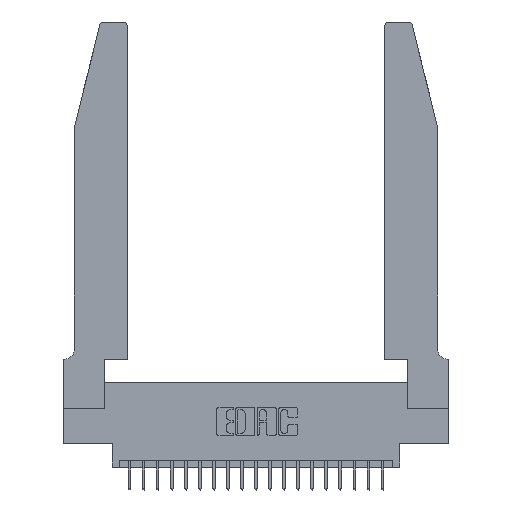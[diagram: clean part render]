
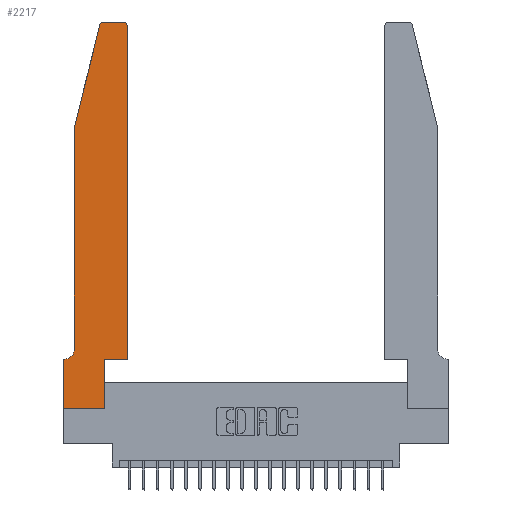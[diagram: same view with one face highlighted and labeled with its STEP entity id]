
A CAD part, top view. The second image highlights one B-rep face of the part: STEP entity #2217.
In plain terms, the highlighted planar face has unit normal (0, 0, 1).
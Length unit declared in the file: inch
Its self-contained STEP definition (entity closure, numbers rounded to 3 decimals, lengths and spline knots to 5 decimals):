
#366 = AXIS2_PLACEMENT_3D ( 'NONE', #951, #13572, #2839 ) ;
#370 = DIRECTION ( 'NONE',  ( 0., 0., 1. ) ) ;
#448 = DIRECTION ( 'NONE',  ( 1., 0., 0. ) ) ;
#672 = AXIS2_PLACEMENT_3D ( 'NONE', #13556, #13503, #14729 ) ;
#673 = CARTESIAN_POINT ( 'NONE',  ( 0.2605, 2.75, 0.37 ) ) ;
#951 = CARTESIAN_POINT ( 'NONE',  ( 0.284, 2.72, 0.37 ) ) ;
#1084 = CARTESIAN_POINT ( 'NONE',  ( 0., 0., 0.37 ) ) ;
#1435 = DIRECTION ( 'NONE',  ( -0.239, -0.971, 0. ) ) ;
#1570 = EDGE_CURVE ( 'NONE', #16445, #22062, #2657, .T. ) ;
#1905 = VERTEX_POINT ( 'NONE', #22014 ) ;
#2094 = VERTEX_POINT ( 'NONE', #20002 ) ;
#2128 = VECTOR ( 'NONE', #18183, 39.37008 ) ;
#2217 = ADVANCED_FACE ( 'NONE', ( #22222 ), #6320, .T. ) ;
#2657 = CIRCLE ( 'NONE', #672, 0.07 ) ;
#2692 = VERTEX_POINT ( 'NONE', #19089 ) ;
#2839 = DIRECTION ( 'NONE',  ( 1., 0., 0. ) ) ;
#3621 = ORIENTED_EDGE ( 'NONE', *, *, #7316, .T. ) ;
#3948 = LINE ( 'NONE', #4196, #8200 ) ;
#4111 = VERTEX_POINT ( 'NONE', #16670 ) ;
#4196 = CARTESIAN_POINT ( 'NONE',  ( 0.0755, 0.35, 0.37 ) ) ;
#4227 = VECTOR ( 'NONE', #13228, 39.37008 ) ;
#4696 = AXIS2_PLACEMENT_3D ( 'NONE', #6292, #370, #448 ) ;
#4809 = VERTEX_POINT ( 'NONE', #1084 ) ;
#5247 = ORIENTED_EDGE ( 'NONE', *, *, #15779, .T. ) ;
#5584 = ORIENTED_EDGE ( 'NONE', *, *, #10149, .T. ) ;
#5890 = DIRECTION ( 'NONE',  ( 0., 0., 1. ) ) ;
#6292 = CARTESIAN_POINT ( 'NONE',  ( 0., 0.35, 0.37 ) ) ;
#6320 = PLANE ( 'NONE',  #4696 ) ;
#6355 = CARTESIAN_POINT ( 'NONE',  ( 0.0755, 2., 0.37 ) ) ;
#6480 = VECTOR ( 'NONE', #13443, 39.37008 ) ;
#6486 = VECTOR ( 'NONE', #14765, 39.37008 ) ;
#6601 = VERTEX_POINT ( 'NONE', #20425 ) ;
#6678 = LINE ( 'NONE', #6851, #20157 ) ;
#6851 = CARTESIAN_POINT ( 'NONE',  ( 0.0755, 2., 0.37 ) ) ;
#7224 = EDGE_CURVE ( 'NONE', #2692, #4111, #15934, .T. ) ;
#7316 = EDGE_CURVE ( 'NONE', #4809, #15855, #13201, .T. ) ;
#7604 = CARTESIAN_POINT ( 'NONE',  ( 0.0055, 0.35, 0.37 ) ) ;
#7618 = CARTESIAN_POINT ( 'NONE',  ( 0.4505, 0.35, 0.37 ) ) ;
#7626 = CARTESIAN_POINT ( 'NONE',  ( 0.2865, 0.35, 0.37 ) ) ;
#7932 = ORIENTED_EDGE ( 'NONE', *, *, #18672, .T. ) ;
#8144 = CARTESIAN_POINT ( 'NONE',  ( 0., 0., 0.37 ) ) ;
#8200 = VECTOR ( 'NONE', #14974, 39.37008 ) ;
#8673 = VECTOR ( 'NONE', #13306, 39.37008 ) ;
#8937 = ORIENTED_EDGE ( 'NONE', *, *, #15851, .T. ) ;
#9087 = VERTEX_POINT ( 'NONE', #16814 ) ;
#9242 = LINE ( 'NONE', #6355, #12320 ) ;
#9661 = CARTESIAN_POINT ( 'NONE',  ( 0., 0., 0.37 ) ) ;
#9767 = EDGE_CURVE ( 'NONE', #6601, #10785, #15601, .T. ) ;
#9821 = EDGE_LOOP ( 'NONE', ( #22665, #20917, #5584, #7932, #10237, #5247, #8937, #3621, #18649, #22607, #12321, #15636 ) ) ;
#10149 = EDGE_CURVE ( 'NONE', #9087, #1905, #6678, .T. ) ;
#10237 = ORIENTED_EDGE ( 'NONE', *, *, #1570, .T. ) ;
#10383 = EDGE_CURVE ( 'NONE', #15855, #2692, #16363, .T. ) ;
#10785 = VERTEX_POINT ( 'NONE', #19156 ) ;
#11072 = VECTOR ( 'NONE', #18880, 39.37008 ) ;
#12320 = VECTOR ( 'NONE', #20446, 39.37008 ) ;
#12321 = ORIENTED_EDGE ( 'NONE', *, *, #13778, .T. ) ;
#13201 = LINE ( 'NONE', #9661, #4227 ) ;
#13228 = DIRECTION ( 'NONE',  ( 1., 0., 0. ) ) ;
#13256 = CARTESIAN_POINT ( 'NONE',  ( 0.0755, 0.42, 0.37 ) ) ;
#13306 = DIRECTION ( 'NONE',  ( -1., 0., 0. ) ) ;
#13443 = DIRECTION ( 'NONE',  ( 0., -1., 0. ) ) ;
#13503 = DIRECTION ( 'NONE',  ( 0., 0., -1. ) ) ;
#13556 = CARTESIAN_POINT ( 'NONE',  ( 0.0055, 0.42, 0.37 ) ) ;
#13572 = DIRECTION ( 'NONE',  ( 0., 0., 1. ) ) ;
#13778 = EDGE_CURVE ( 'NONE', #4111, #6601, #20346, .T. ) ;
#14729 = DIRECTION ( 'NONE',  ( -1., 0., 0. ) ) ;
#14765 = DIRECTION ( 'NONE',  ( 1., 0., 0. ) ) ;
#14974 = DIRECTION ( 'NONE',  ( -1., 0., 0. ) ) ;
#15601 = CIRCLE ( 'NONE', #19499, 0.03 ) ;
#15636 = ORIENTED_EDGE ( 'NONE', *, *, #9767, .T. ) ;
#15779 = EDGE_CURVE ( 'NONE', #22062, #22305, #3948, .T. ) ;
#15851 = EDGE_CURVE ( 'NONE', #22305, #4809, #16458, .T. ) ;
#15855 = VERTEX_POINT ( 'NONE', #22141 ) ;
#15934 = LINE ( 'NONE', #7618, #6486 ) ;
#16363 = LINE ( 'NONE', #7626, #2128 ) ;
#16445 = VERTEX_POINT ( 'NONE', #13256 ) ;
#16458 = LINE ( 'NONE', #8144, #6480 ) ;
#16537 = CARTESIAN_POINT ( 'NONE',  ( 0.4205, 2.72, 0.37 ) ) ;
#16670 = CARTESIAN_POINT ( 'NONE',  ( 0.4505, 0.35, 0.37 ) ) ;
#16814 = CARTESIAN_POINT ( 'NONE',  ( 0.25487, 2.72718, 0.37 ) ) ;
#17148 = CARTESIAN_POINT ( 'NONE',  ( 0.4505, 0.35, 0.37 ) ) ;
#18183 = DIRECTION ( 'NONE',  ( 0., 1., 0. ) ) ;
#18286 = DIRECTION ( 'NONE',  ( 1., 0., 0. ) ) ;
#18649 = ORIENTED_EDGE ( 'NONE', *, *, #10383, .T. ) ;
#18672 = EDGE_CURVE ( 'NONE', #1905, #16445, #9242, .T. ) ;
#18880 = DIRECTION ( 'NONE',  ( 0., 1., 0. ) ) ;
#19089 = CARTESIAN_POINT ( 'NONE',  ( 0.2865, 0.35, 0.37 ) ) ;
#19107 = EDGE_CURVE ( 'NONE', #10785, #2094, #22054, .T. ) ;
#19156 = CARTESIAN_POINT ( 'NONE',  ( 0.4205, 2.75, 0.37 ) ) ;
#19499 = AXIS2_PLACEMENT_3D ( 'NONE', #16537, #5890, #18286 ) ;
#20002 = CARTESIAN_POINT ( 'NONE',  ( 0.284, 2.75, 0.37 ) ) ;
#20157 = VECTOR ( 'NONE', #1435, 39.37008 ) ;
#20346 = LINE ( 'NONE', #17148, #11072 ) ;
#20418 = CARTESIAN_POINT ( 'NONE',  ( 0., 0.35, 0.37 ) ) ;
#20425 = CARTESIAN_POINT ( 'NONE',  ( 0.4505, 2.72, 0.37 ) ) ;
#20446 = DIRECTION ( 'NONE',  ( 0., -1., 0. ) ) ;
#20917 = ORIENTED_EDGE ( 'NONE', *, *, #21181, .T. ) ;
#21139 = CIRCLE ( 'NONE', #366, 0.03 ) ;
#21181 = EDGE_CURVE ( 'NONE', #2094, #9087, #21139, .T. ) ;
#22014 = CARTESIAN_POINT ( 'NONE',  ( 0.0755, 2., 0.37 ) ) ;
#22054 = LINE ( 'NONE', #673, #8673 ) ;
#22062 = VERTEX_POINT ( 'NONE', #7604 ) ;
#22141 = CARTESIAN_POINT ( 'NONE',  ( 0.2865, 0., 0.37 ) ) ;
#22222 = FACE_OUTER_BOUND ( 'NONE', #9821, .T. ) ;
#22305 = VERTEX_POINT ( 'NONE', #20418 ) ;
#22607 = ORIENTED_EDGE ( 'NONE', *, *, #7224, .T. ) ;
#22665 = ORIENTED_EDGE ( 'NONE', *, *, #19107, .T. ) ;
